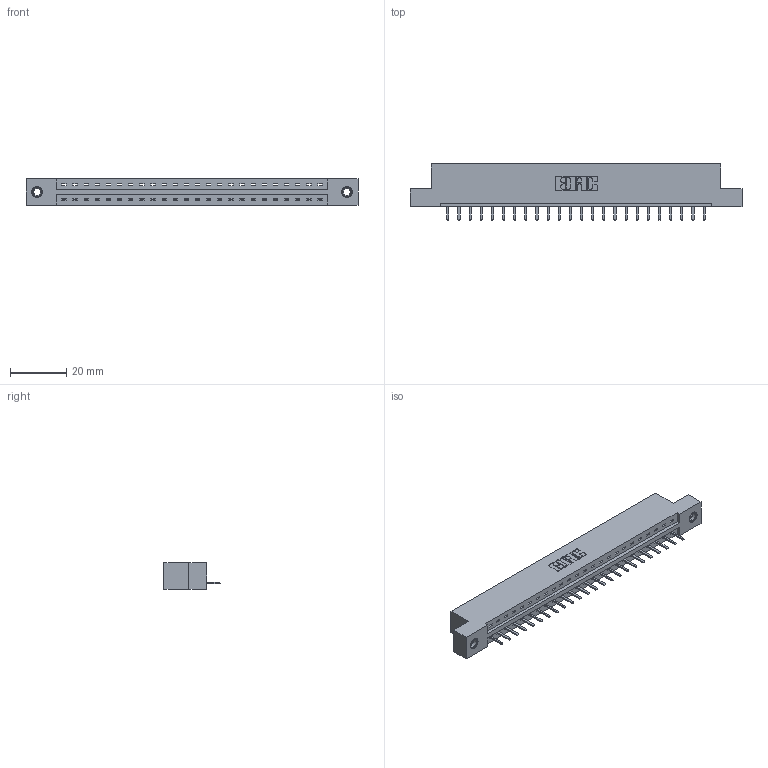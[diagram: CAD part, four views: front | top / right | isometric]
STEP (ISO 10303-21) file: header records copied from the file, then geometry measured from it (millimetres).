
FILE_DESCRIPTION (( 'STEP AP203' ), '1' );
FILE_NAME ('337-024-520-107.STEP', '2018-08-05T18:19:32', ( '' ), ( '' ), 'SwSTEP 2.0', 'SolidWorks 2016', '' );
FILE_SCHEMA (( 'CONFIG_CONTROL_DESIGN' ));
Length unit declared in the file: inch
Products named in the file (4): 337 Part_Flush Mounting Lugs - 0.156 Dia-TI; 345-292-001_345-293-120; 345-250-001_345-250-005-103; 337-024-520-107
Assembly tree (27 placements, depth 2):
  337-024-520-107
    337 Part_Flush Mounting Lugs - 0.156 Dia-TI
    345-292-001_345-293-120  x24
    345-250-001_345-250-005-103  x2
Bounding box: 118.11 x 20.02 x 9.4 mm (x, y, z)
Volume: 11967.7 mm3; surface area: 12059.5 mm2
Topology: 27 solids, 27 shells, 1758 faces, 5151 edges, 3362 vertices
Faces by surface type: plane 1254, cylinder 488, cone 12, torus 4
Entity records: 21468 total; most frequent: CARTESIAN_POINT 3729, ORIENTED_EDGE 3670, DIRECTION 3197, EDGE_CURVE 1835, LINE 1683, VECTOR 1683, VERTEX_POINT 1216, AXIS2_PLACEMENT_3D 757
